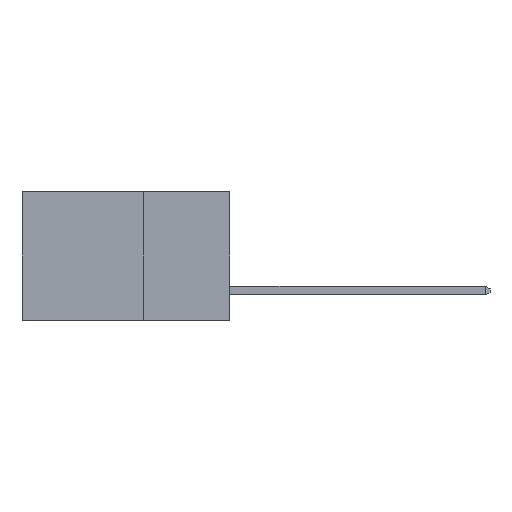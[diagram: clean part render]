
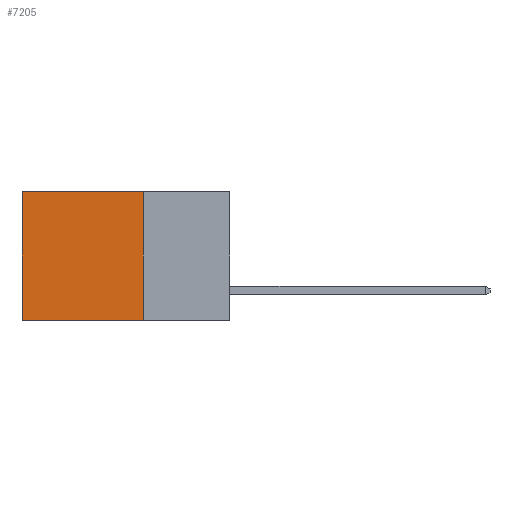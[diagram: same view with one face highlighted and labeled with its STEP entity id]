
A CAD part, left-side view. The second image highlights one B-rep face of the part: STEP entity #7205.
In plain terms, the highlighted planar face has unit normal (-1, 0, 0).
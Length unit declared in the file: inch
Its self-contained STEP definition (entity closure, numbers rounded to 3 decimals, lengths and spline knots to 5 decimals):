
#2004 = VERTEX_POINT ( 'NONE', #19442 ) ;
#2678 = VECTOR ( 'NONE', #16892, 39.37008 ) ;
#2952 = CARTESIAN_POINT ( 'NONE',  ( 0.298, 0.25, 0. ) ) ;
#4235 = EDGE_CURVE ( 'NONE', #18307, #2004, #16307, .T. ) ;
#5273 = CARTESIAN_POINT ( 'NONE',  ( 0.298, 0.6, 0. ) ) ;
#5407 = ORIENTED_EDGE ( 'NONE', *, *, #4235, .F. ) ;
#6425 = VERTEX_POINT ( 'NONE', #9306 ) ;
#6586 = ORIENTED_EDGE ( 'NONE', *, *, #10838, .T. ) ;
#7113 = DIRECTION ( 'NONE',  ( 0., 0., -1. ) ) ;
#7205 = ADVANCED_FACE ( 'NONE', ( #16633 ), #24337, .F. ) ;
#7651 = CARTESIAN_POINT ( 'NONE',  ( 0.298, 0.25, -0.37 ) ) ;
#8857 = VECTOR ( 'NONE', #7113, 39.37008 ) ;
#8919 = EDGE_CURVE ( 'NONE', #6425, #18307, #15392, .T. ) ;
#9146 = CARTESIAN_POINT ( 'NONE',  ( 0.298, 0.25, -0.37 ) ) ;
#9230 = EDGE_LOOP ( 'NONE', ( #6586, #5407, #15364, #19277 ) ) ;
#9306 = CARTESIAN_POINT ( 'NONE',  ( 0.298, 0.25, 0. ) ) ;
#10560 = LINE ( 'NONE', #2952, #29283 ) ;
#10838 = EDGE_CURVE ( 'NONE', #27257, #2004, #16515, .T. ) ;
#14376 = CARTESIAN_POINT ( 'NONE',  ( 0.298, 0.6, 0. ) ) ;
#15364 = ORIENTED_EDGE ( 'NONE', *, *, #8919, .F. ) ;
#15392 = LINE ( 'NONE', #17372, #8857 ) ;
#16307 = LINE ( 'NONE', #9146, #28489 ) ;
#16515 = LINE ( 'NONE', #14376, #2678 ) ;
#16633 = FACE_OUTER_BOUND ( 'NONE', #9230, .T. ) ;
#16892 = DIRECTION ( 'NONE',  ( 0., 0., -1. ) ) ;
#17372 = CARTESIAN_POINT ( 'NONE',  ( 0.298, 0.25, 0. ) ) ;
#18307 = VERTEX_POINT ( 'NONE', #7651 ) ;
#19277 = ORIENTED_EDGE ( 'NONE', *, *, #21316, .T. ) ;
#19442 = CARTESIAN_POINT ( 'NONE',  ( 0.298, 0.6, -0.37 ) ) ;
#21316 = EDGE_CURVE ( 'NONE', #6425, #27257, #10560, .T. ) ;
#22060 = DIRECTION ( 'NONE',  ( 0., 1., 0. ) ) ;
#24001 = DIRECTION ( 'NONE',  ( 0., 0., -1. ) ) ;
#24103 = DIRECTION ( 'NONE',  ( 1., 0., 0. ) ) ;
#24337 = PLANE ( 'NONE',  #25147 ) ;
#24983 = DIRECTION ( 'NONE',  ( 0., 1., 0. ) ) ;
#25147 = AXIS2_PLACEMENT_3D ( 'NONE', #28955, #24103, #24001 ) ;
#27257 = VERTEX_POINT ( 'NONE', #5273 ) ;
#28489 = VECTOR ( 'NONE', #22060, 39.37008 ) ;
#28955 = CARTESIAN_POINT ( 'NONE',  ( 0.298, 0.25, 0. ) ) ;
#29283 = VECTOR ( 'NONE', #24983, 39.37008 ) ;
